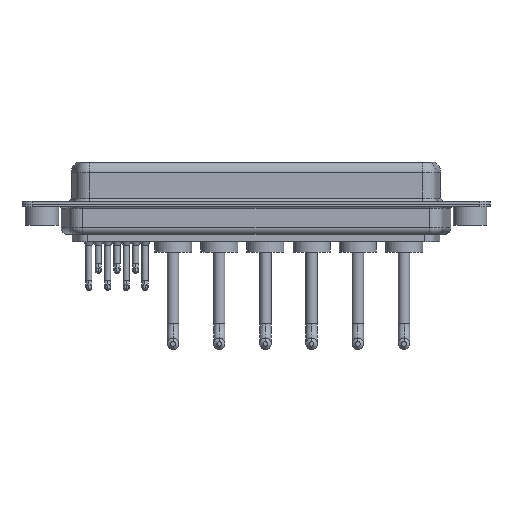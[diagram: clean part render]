
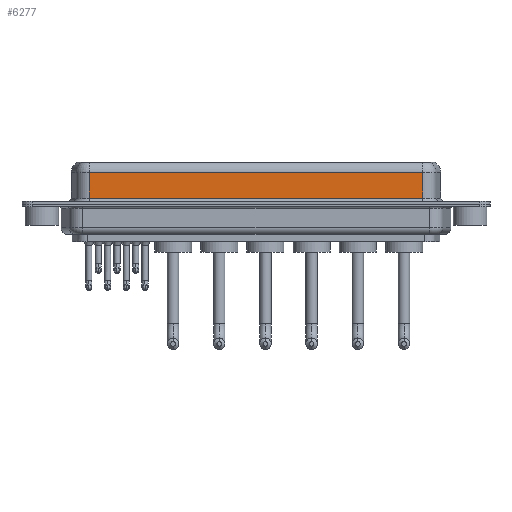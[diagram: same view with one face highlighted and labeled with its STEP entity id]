
A CAD part, front view. The second image highlights one B-rep face of the part: STEP entity #6277.
In plain terms, the highlighted planar face has unit normal (0, -1, 0).
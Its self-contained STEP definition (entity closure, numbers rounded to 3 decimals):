
#103 = DIRECTION ( 'NONE',  ( 0., 0., -1. ) ) ;
#1601 = CARTESIAN_POINT ( 'NONE',  ( 7.038, -3.95, 6.4 ) ) ;
#1889 = VERTEX_POINT ( 'NONE', #12456 ) ;
#2023 = LINE ( 'NONE', #7766, #6632 ) ;
#3019 = EDGE_CURVE ( 'NONE', #11534, #15501, #2023, .T. ) ;
#4870 = LINE ( 'NONE', #11770, #14323 ) ;
#5475 = LINE ( 'NONE', #8548, #7101 ) ;
#6277 = ADVANCED_FACE ( 'NONE', ( #13571 ), #11887, .F. ) ;
#6367 = ORIENTED_EDGE ( 'NONE', *, *, #15711, .T. ) ;
#6453 = DIRECTION ( 'NONE',  ( 0., 0., -1. ) ) ;
#6632 = VECTOR ( 'NONE', #6453, 1000. ) ;
#7101 = VECTOR ( 'NONE', #8467, 1000. ) ;
#7766 = CARTESIAN_POINT ( 'NONE',  ( 56.462, -3.95, 6.4 ) ) ;
#7771 = ORIENTED_EDGE ( 'NONE', *, *, #3019, .F. ) ;
#7800 = CARTESIAN_POINT ( 'NONE',  ( 56.462, -3.95, 6.4 ) ) ;
#8182 = AXIS2_PLACEMENT_3D ( 'NONE', #7800, #11976, #14873 ) ;
#8467 = DIRECTION ( 'NONE',  ( -1., 0., 0. ) ) ;
#8548 = CARTESIAN_POINT ( 'NONE',  ( 56.462, -3.95, 4.65 ) ) ;
#9835 = VECTOR ( 'NONE', #103, 1000. ) ;
#9962 = CARTESIAN_POINT ( 'NONE',  ( 56.462, -3.95, 4.65 ) ) ;
#10939 = VERTEX_POINT ( 'NONE', #13552 ) ;
#11504 = EDGE_CURVE ( 'NONE', #11534, #1889, #5475, .T. ) ;
#11534 = VERTEX_POINT ( 'NONE', #9962 ) ;
#11770 = CARTESIAN_POINT ( 'NONE',  ( 56.462, -3.95, 0.9 ) ) ;
#11887 = PLANE ( 'NONE',  #8182 ) ;
#11976 = DIRECTION ( 'NONE',  ( 0., 1., 0. ) ) ;
#12456 = CARTESIAN_POINT ( 'NONE',  ( 7.038, -3.95, 4.65 ) ) ;
#12890 = CARTESIAN_POINT ( 'NONE',  ( 56.462, -3.95, 0.9 ) ) ;
#13552 = CARTESIAN_POINT ( 'NONE',  ( 7.038, -3.95, 0.9 ) ) ;
#13571 = FACE_OUTER_BOUND ( 'NONE', #14782, .T. ) ;
#14323 = VECTOR ( 'NONE', #17547, 1000. ) ;
#14707 = EDGE_CURVE ( 'NONE', #1889, #10939, #15629, .T. ) ;
#14782 = EDGE_LOOP ( 'NONE', ( #7771, #16329, #17842, #6367 ) ) ;
#14873 = DIRECTION ( 'NONE',  ( 0., 0., 1. ) ) ;
#15501 = VERTEX_POINT ( 'NONE', #12890 ) ;
#15629 = LINE ( 'NONE', #1601, #9835 ) ;
#15711 = EDGE_CURVE ( 'NONE', #10939, #15501, #4870, .T. ) ;
#16329 = ORIENTED_EDGE ( 'NONE', *, *, #11504, .T. ) ;
#17547 = DIRECTION ( 'NONE',  ( 1., 0., 0. ) ) ;
#17842 = ORIENTED_EDGE ( 'NONE', *, *, #14707, .T. ) ;
